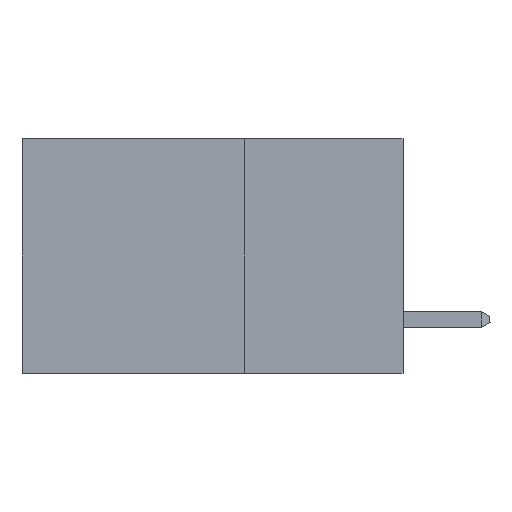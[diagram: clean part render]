
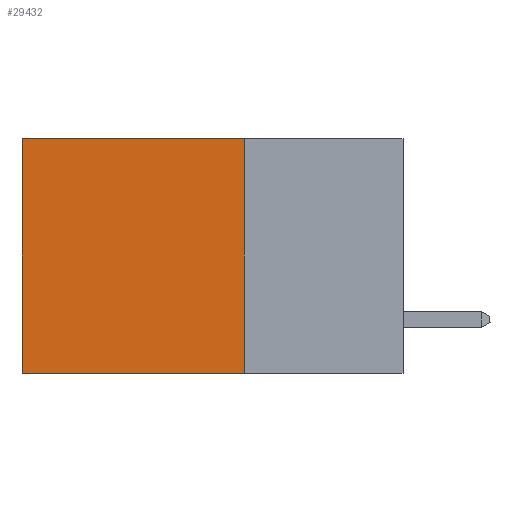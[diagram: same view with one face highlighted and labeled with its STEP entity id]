
A CAD part, left-side view. The second image highlights one B-rep face of the part: STEP entity #29432.
In plain terms, the highlighted planar face has unit normal (-1, 0, 0).
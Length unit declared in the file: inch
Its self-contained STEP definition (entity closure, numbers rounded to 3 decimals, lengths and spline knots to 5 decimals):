
#304 = LINE ( 'NONE', #1795, #37240 ) ;
#1795 = CARTESIAN_POINT ( 'NONE',  ( 0.2875, 0.6, 0. ) ) ;
#1953 = EDGE_CURVE ( 'NONE', #11671, #8471, #36082, .T. ) ;
#2674 = ORIENTED_EDGE ( 'NONE', *, *, #25686, .T. ) ;
#2917 = DIRECTION ( 'NONE',  ( 1., 0., 0. ) ) ;
#3384 = LINE ( 'NONE', #29098, #27165 ) ;
#6243 = LINE ( 'NONE', #13693, #16372 ) ;
#7122 = DIRECTION ( 'NONE',  ( 0., 0., -1. ) ) ;
#7208 = EDGE_LOOP ( 'NONE', ( #24138, #19891, #20472, #2674 ) ) ;
#7534 = CARTESIAN_POINT ( 'NONE',  ( 0.2875, 0.6, 0. ) ) ;
#7636 = DIRECTION ( 'NONE',  ( 0., 0., -1. ) ) ;
#8471 = VERTEX_POINT ( 'NONE', #16891 ) ;
#9145 = PLANE ( 'NONE',  #29743 ) ;
#11671 = VERTEX_POINT ( 'NONE', #13339 ) ;
#13339 = CARTESIAN_POINT ( 'NONE',  ( 0.2875, 0.25, 0. ) ) ;
#13693 = CARTESIAN_POINT ( 'NONE',  ( 0.2875, 0.25, 0. ) ) ;
#14908 = DIRECTION ( 'NONE',  ( 0., 1., 0. ) ) ;
#16372 = VECTOR ( 'NONE', #16521, 39.37008 ) ;
#16521 = DIRECTION ( 'NONE',  ( 0., 1., 0. ) ) ;
#16891 = CARTESIAN_POINT ( 'NONE',  ( 0.2875, 0.25, -0.37 ) ) ;
#17643 = VERTEX_POINT ( 'NONE', #36604 ) ;
#19047 = CARTESIAN_POINT ( 'NONE',  ( 0.2875, 0.25, 0. ) ) ;
#19891 = ORIENTED_EDGE ( 'NONE', *, *, #24757, .F. ) ;
#20472 = ORIENTED_EDGE ( 'NONE', *, *, #1953, .F. ) ;
#20607 = VECTOR ( 'NONE', #7122, 39.37008 ) ;
#20730 = DIRECTION ( 'NONE',  ( 0., 0., -1. ) ) ;
#24138 = ORIENTED_EDGE ( 'NONE', *, *, #37249, .T. ) ;
#24757 = EDGE_CURVE ( 'NONE', #8471, #17643, #3384, .T. ) ;
#25686 = EDGE_CURVE ( 'NONE', #11671, #29196, #6243, .T. ) ;
#27165 = VECTOR ( 'NONE', #14908, 39.37008 ) ;
#29098 = CARTESIAN_POINT ( 'NONE',  ( 0.2875, 0.25, -0.37 ) ) ;
#29196 = VERTEX_POINT ( 'NONE', #7534 ) ;
#29432 = ADVANCED_FACE ( 'NONE', ( #34355 ), #9145, .F. ) ;
#29743 = AXIS2_PLACEMENT_3D ( 'NONE', #34992, #2917, #20730 ) ;
#34355 = FACE_OUTER_BOUND ( 'NONE', #7208, .T. ) ;
#34992 = CARTESIAN_POINT ( 'NONE',  ( 0.2875, 0.25, 0. ) ) ;
#36082 = LINE ( 'NONE', #19047, #20607 ) ;
#36604 = CARTESIAN_POINT ( 'NONE',  ( 0.2875, 0.6, -0.37 ) ) ;
#37240 = VECTOR ( 'NONE', #7636, 39.37008 ) ;
#37249 = EDGE_CURVE ( 'NONE', #29196, #17643, #304, .T. ) ;
